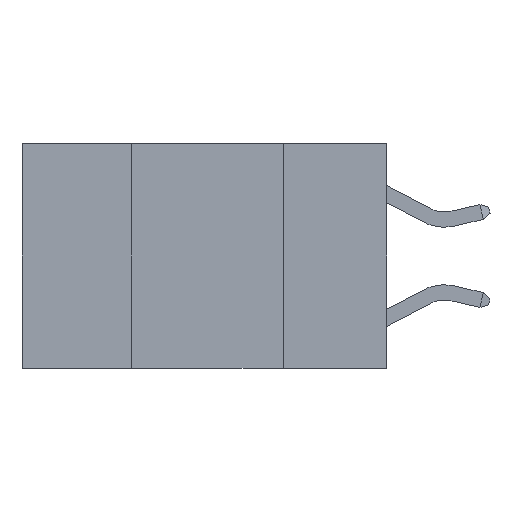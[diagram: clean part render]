
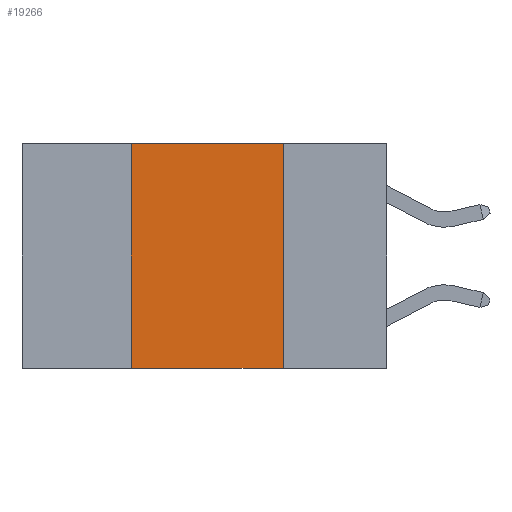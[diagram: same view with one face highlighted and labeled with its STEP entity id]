
A CAD part, left-side view. The second image highlights one B-rep face of the part: STEP entity #19266.
In plain terms, the highlighted planar face has unit normal (-1, 0, 0).
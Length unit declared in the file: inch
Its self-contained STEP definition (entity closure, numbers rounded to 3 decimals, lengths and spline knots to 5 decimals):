
#108 = ORIENTED_EDGE ( 'NONE', *, *, #3786, .F. ) ;
#310 = CARTESIAN_POINT ( 'NONE',  ( 0., 0.6, 0. ) ) ;
#505 = EDGE_CURVE ( 'NONE', #9930, #19166, #10105, .T. ) ;
#1642 = DIRECTION ( 'NONE',  ( 0., 0., -1. ) ) ;
#2599 = VECTOR ( 'NONE', #1642, 39.37008 ) ;
#2966 = CARTESIAN_POINT ( 'NONE',  ( 0., 0.6, -0.37 ) ) ;
#3786 = EDGE_CURVE ( 'NONE', #9930, #17006, #14450, .T. ) ;
#4239 = PLANE ( 'NONE',  #22531 ) ;
#4355 = FACE_OUTER_BOUND ( 'NONE', #12429, .T. ) ;
#4878 = VECTOR ( 'NONE', #18266, 39.37008 ) ;
#5095 = CARTESIAN_POINT ( 'NONE',  ( 0., 0.17, 0. ) ) ;
#5130 = ORIENTED_EDGE ( 'NONE', *, *, #17322, .F. ) ;
#5299 = CARTESIAN_POINT ( 'NONE',  ( 0., 0.42, -0.37 ) ) ;
#6350 = CARTESIAN_POINT ( 'NONE',  ( 0., 0.17, 0. ) ) ;
#7709 = DIRECTION ( 'NONE',  ( 1., 0., 0. ) ) ;
#8478 = VERTEX_POINT ( 'NONE', #6350 ) ;
#9930 = VERTEX_POINT ( 'NONE', #5299 ) ;
#10105 = LINE ( 'NONE', #2966, #14911 ) ;
#10400 = LINE ( 'NONE', #5095, #2599 ) ;
#10501 = VECTOR ( 'NONE', #19619, 39.37008 ) ;
#11411 = CARTESIAN_POINT ( 'NONE',  ( 0., 0.6, 0. ) ) ;
#12429 = EDGE_LOOP ( 'NONE', ( #5130, #18398, #108, #20865 ) ) ;
#14450 = LINE ( 'NONE', #21002, #10501 ) ;
#14489 = LINE ( 'NONE', #310, #4878 ) ;
#14911 = VECTOR ( 'NONE', #17118, 39.37008 ) ;
#17006 = VERTEX_POINT ( 'NONE', #18235 ) ;
#17118 = DIRECTION ( 'NONE',  ( 0., -1., 0. ) ) ;
#17322 = EDGE_CURVE ( 'NONE', #8478, #19166, #10400, .T. ) ;
#18235 = CARTESIAN_POINT ( 'NONE',  ( 0., 0.42, 0. ) ) ;
#18266 = DIRECTION ( 'NONE',  ( 0., -1., 0. ) ) ;
#18398 = ORIENTED_EDGE ( 'NONE', *, *, #19781, .F. ) ;
#19166 = VERTEX_POINT ( 'NONE', #19572 ) ;
#19266 = ADVANCED_FACE ( 'NONE', ( #4355 ), #4239, .F. ) ;
#19572 = CARTESIAN_POINT ( 'NONE',  ( 0., 0.17, -0.37 ) ) ;
#19619 = DIRECTION ( 'NONE',  ( 0., 0., 1. ) ) ;
#19781 = EDGE_CURVE ( 'NONE', #17006, #8478, #14489, .T. ) ;
#20865 = ORIENTED_EDGE ( 'NONE', *, *, #505, .T. ) ;
#21002 = CARTESIAN_POINT ( 'NONE',  ( 0., 0.42, 0. ) ) ;
#21545 = DIRECTION ( 'NONE',  ( 0., 0., -1. ) ) ;
#22531 = AXIS2_PLACEMENT_3D ( 'NONE', #11411, #7709, #21545 ) ;
